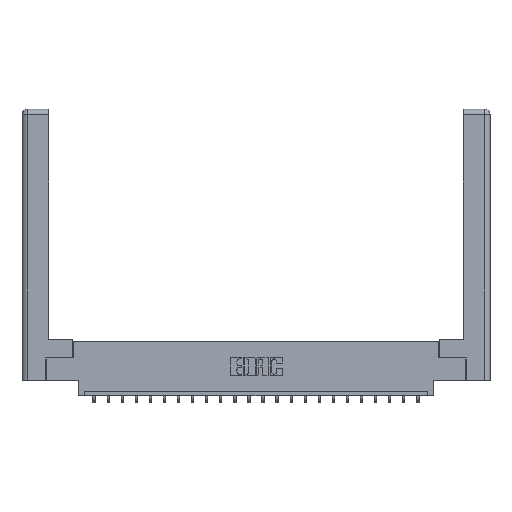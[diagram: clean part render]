
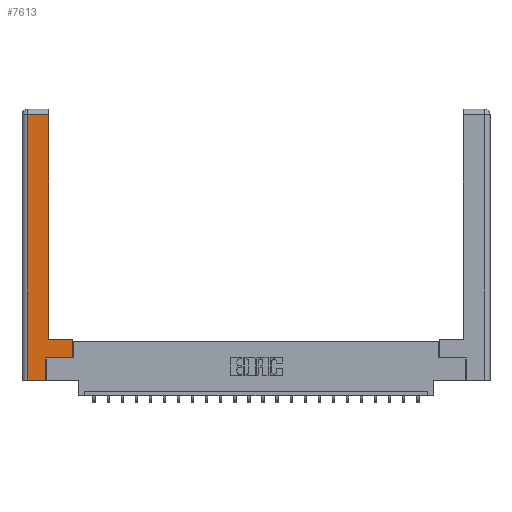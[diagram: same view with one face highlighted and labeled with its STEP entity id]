
A CAD part, top view. The second image highlights one B-rep face of the part: STEP entity #7613.
In plain terms, the highlighted planar face has unit normal (0, 0, 1).
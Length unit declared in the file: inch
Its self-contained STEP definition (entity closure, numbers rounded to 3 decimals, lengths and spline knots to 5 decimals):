
#506 = CARTESIAN_POINT ( 'NONE',  ( 0.295, 2.94, 0. ) ) ;
#572 = VERTEX_POINT ( 'NONE', #11618 ) ;
#593 = DIRECTION ( 'NONE',  ( -1., 0., 0. ) ) ;
#1104 = ORIENTED_EDGE ( 'NONE', *, *, #18696, .T. ) ;
#1265 = LINE ( 'NONE', #2970, #9640 ) ;
#1424 = ORIENTED_EDGE ( 'NONE', *, *, #13576, .T. ) ;
#1663 = DIRECTION ( 'NONE',  ( 1., 0., 0. ) ) ;
#2044 = LINE ( 'NONE', #5803, #14812 ) ;
#2469 = VERTEX_POINT ( 'NONE', #7784 ) ;
#2807 = DIRECTION ( 'NONE',  ( 0., 1., 0. ) ) ;
#2970 = CARTESIAN_POINT ( 'NONE',  ( 0.295, 3., 0. ) ) ;
#3103 = CARTESIAN_POINT ( 'NONE',  ( 0.0615, 0., 0. ) ) ;
#3530 = VECTOR ( 'NONE', #15486, 39.37008 ) ;
#3744 = LINE ( 'NONE', #17133, #9862 ) ;
#4544 = VECTOR ( 'NONE', #1663, 39.37008 ) ;
#5019 = VERTEX_POINT ( 'NONE', #20471 ) ;
#5689 = DIRECTION ( 'NONE',  ( -1., 0., 0. ) ) ;
#5803 = CARTESIAN_POINT ( 'NONE',  ( 0.0615, 2.94, 0. ) ) ;
#5830 = VERTEX_POINT ( 'NONE', #6266 ) ;
#6266 = CARTESIAN_POINT ( 'NONE',  ( 0.0615, 2.94, 0. ) ) ;
#6448 = CARTESIAN_POINT ( 'NONE',  ( 0.565, 0.245, 0. ) ) ;
#6469 = VERTEX_POINT ( 'NONE', #15000 ) ;
#6628 = ORIENTED_EDGE ( 'NONE', *, *, #17151, .T. ) ;
#7143 = CARTESIAN_POINT ( 'NONE',  ( 0., 0., 0. ) ) ;
#7613 = ADVANCED_FACE ( 'NONE', ( #11134 ), #21216, .F. ) ;
#7784 = CARTESIAN_POINT ( 'NONE',  ( 0.265, 0.245, 0. ) ) ;
#7998 = LINE ( 'NONE', #3103, #3530 ) ;
#8228 = DIRECTION ( 'NONE',  ( 0., 1., 0. ) ) ;
#8676 = VERTEX_POINT ( 'NONE', #13975 ) ;
#9259 = LINE ( 'NONE', #22945, #4544 ) ;
#9640 = VECTOR ( 'NONE', #2807, 39.37008 ) ;
#9729 = ORIENTED_EDGE ( 'NONE', *, *, #22014, .T. ) ;
#9856 = ORIENTED_EDGE ( 'NONE', *, *, #10113, .T. ) ;
#9862 = VECTOR ( 'NONE', #10354, 39.37008 ) ;
#9890 = ORIENTED_EDGE ( 'NONE', *, *, #18980, .T. ) ;
#9969 = VECTOR ( 'NONE', #22270, 39.37008 ) ;
#10043 = AXIS2_PLACEMENT_3D ( 'NONE', #7143, #19882, #5689 ) ;
#10113 = EDGE_CURVE ( 'NONE', #572, #6469, #3744, .T. ) ;
#10213 = ORIENTED_EDGE ( 'NONE', *, *, #10946, .T. ) ;
#10354 = DIRECTION ( 'NONE',  ( -1., 0., 0. ) ) ;
#10946 = EDGE_CURVE ( 'NONE', #5830, #5019, #7998, .T. ) ;
#11134 = FACE_OUTER_BOUND ( 'NONE', #18793, .T. ) ;
#11618 = CARTESIAN_POINT ( 'NONE',  ( 0.565, 0.45, 0. ) ) ;
#11701 = CARTESIAN_POINT ( 'NONE',  ( 0.565, 0.245, 0. ) ) ;
#13183 = CARTESIAN_POINT ( 'NONE',  ( 0.265, 0.245, 0. ) ) ;
#13435 = VERTEX_POINT ( 'NONE', #6448 ) ;
#13552 = LINE ( 'NONE', #13183, #9969 ) ;
#13576 = EDGE_CURVE ( 'NONE', #2469, #13435, #19370, .T. ) ;
#13975 = CARTESIAN_POINT ( 'NONE',  ( 0.265, 0., 0. ) ) ;
#14638 = VECTOR ( 'NONE', #15240, 39.37008 ) ;
#14812 = VECTOR ( 'NONE', #593, 39.37008 ) ;
#15000 = CARTESIAN_POINT ( 'NONE',  ( 0.295, 0.45, 0. ) ) ;
#15240 = DIRECTION ( 'NONE',  ( 1., 0., 0. ) ) ;
#15486 = DIRECTION ( 'NONE',  ( 0., -1., 0. ) ) ;
#15789 = EDGE_CURVE ( 'NONE', #5019, #8676, #9259, .T. ) ;
#16459 = LINE ( 'NONE', #17234, #19265 ) ;
#17133 = CARTESIAN_POINT ( 'NONE',  ( 0.295, 0.45, 0. ) ) ;
#17151 = EDGE_CURVE ( 'NONE', #6469, #20549, #1265, .T. ) ;
#17234 = CARTESIAN_POINT ( 'NONE',  ( 0.565, 0.45, 0. ) ) ;
#17730 = ORIENTED_EDGE ( 'NONE', *, *, #15789, .T. ) ;
#18696 = EDGE_CURVE ( 'NONE', #20549, #5830, #2044, .T. ) ;
#18793 = EDGE_LOOP ( 'NONE', ( #6628, #1104, #10213, #17730, #9729, #1424, #9890, #9856 ) ) ;
#18980 = EDGE_CURVE ( 'NONE', #13435, #572, #16459, .T. ) ;
#19265 = VECTOR ( 'NONE', #8228, 39.37008 ) ;
#19370 = LINE ( 'NONE', #11701, #14638 ) ;
#19882 = DIRECTION ( 'NONE',  ( 0., 0., -1. ) ) ;
#20471 = CARTESIAN_POINT ( 'NONE',  ( 0.0615, 0., 0. ) ) ;
#20549 = VERTEX_POINT ( 'NONE', #506 ) ;
#21216 = PLANE ( 'NONE',  #10043 ) ;
#22014 = EDGE_CURVE ( 'NONE', #8676, #2469, #13552, .T. ) ;
#22270 = DIRECTION ( 'NONE',  ( 0., 1., 0. ) ) ;
#22945 = CARTESIAN_POINT ( 'NONE',  ( 0.265, 0., 0. ) ) ;
